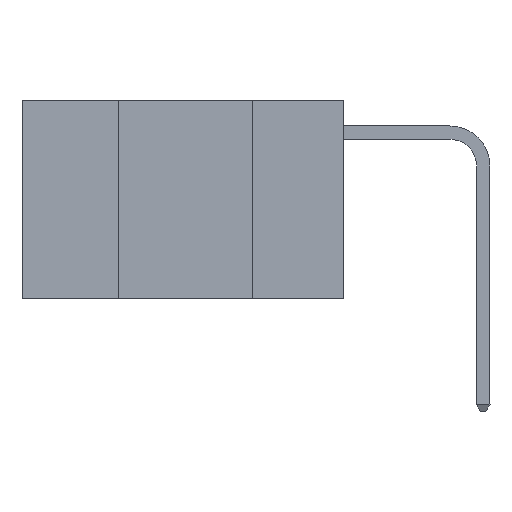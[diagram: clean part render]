
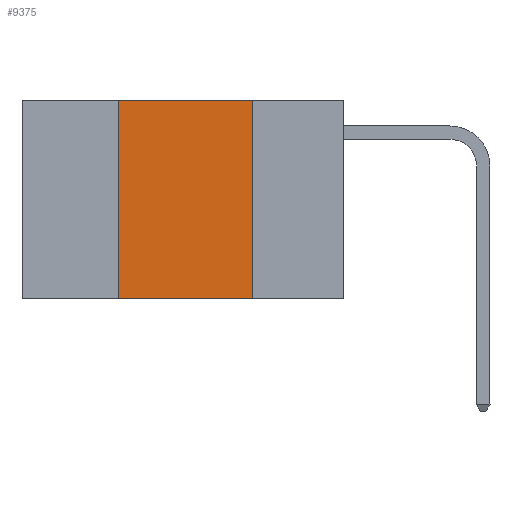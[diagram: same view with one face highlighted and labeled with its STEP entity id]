
A CAD part, left-side view. The second image highlights one B-rep face of the part: STEP entity #9375.
In plain terms, the highlighted planar face has unit normal (-1, 0, 0).
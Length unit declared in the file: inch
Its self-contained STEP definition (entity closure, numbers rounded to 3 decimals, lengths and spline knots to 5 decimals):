
#292 = ORIENTED_EDGE ( 'NONE', *, *, #7636, .T. ) ;
#629 = LINE ( 'NONE', #2177, #1024 ) ;
#890 = VECTOR ( 'NONE', #2272, 39.37008 ) ;
#930 = CARTESIAN_POINT ( 'NONE',  ( 0., 0.6, -0.37 ) ) ;
#1024 = VECTOR ( 'NONE', #1471, 39.37008 ) ;
#1281 = AXIS2_PLACEMENT_3D ( 'NONE', #4069, #4628, #7953 ) ;
#1471 = DIRECTION ( 'NONE',  ( 0., 0., 1. ) ) ;
#2177 = CARTESIAN_POINT ( 'NONE',  ( 0., 0.42, 0. ) ) ;
#2267 = VERTEX_POINT ( 'NONE', #10170 ) ;
#2272 = DIRECTION ( 'NONE',  ( 0., -1., 0. ) ) ;
#2513 = DIRECTION ( 'NONE',  ( 0., -1., 0. ) ) ;
#2635 = VERTEX_POINT ( 'NONE', #8420 ) ;
#2984 = VERTEX_POINT ( 'NONE', #5144 ) ;
#3816 = LINE ( 'NONE', #7000, #9246 ) ;
#4013 = FACE_OUTER_BOUND ( 'NONE', #5321, .T. ) ;
#4069 = CARTESIAN_POINT ( 'NONE',  ( 0., 0.6, 0. ) ) ;
#4628 = DIRECTION ( 'NONE',  ( 1., 0., 0. ) ) ;
#4758 = CARTESIAN_POINT ( 'NONE',  ( 0., 0.6, 0. ) ) ;
#5144 = CARTESIAN_POINT ( 'NONE',  ( 0., 0.17, 0. ) ) ;
#5321 = EDGE_LOOP ( 'NONE', ( #7345, #5951, #9402, #292 ) ) ;
#5951 = ORIENTED_EDGE ( 'NONE', *, *, #6680, .F. ) ;
#6680 = EDGE_CURVE ( 'NONE', #2267, #2984, #7622, .T. ) ;
#7000 = CARTESIAN_POINT ( 'NONE',  ( 0., 0.17, 0. ) ) ;
#7233 = PLANE ( 'NONE',  #1281 ) ;
#7345 = ORIENTED_EDGE ( 'NONE', *, *, #7482, .F. ) ;
#7482 = EDGE_CURVE ( 'NONE', #2984, #9340, #3816, .T. ) ;
#7578 = VECTOR ( 'NONE', #2513, 39.37008 ) ;
#7622 = LINE ( 'NONE', #4758, #890 ) ;
#7636 = EDGE_CURVE ( 'NONE', #2635, #9340, #9675, .T. ) ;
#7850 = EDGE_CURVE ( 'NONE', #2635, #2267, #629, .T. ) ;
#7953 = DIRECTION ( 'NONE',  ( 0., 0., -1. ) ) ;
#8420 = CARTESIAN_POINT ( 'NONE',  ( 0., 0.42, -0.37 ) ) ;
#8799 = CARTESIAN_POINT ( 'NONE',  ( 0., 0.17, -0.37 ) ) ;
#9246 = VECTOR ( 'NONE', #10047, 39.37008 ) ;
#9340 = VERTEX_POINT ( 'NONE', #8799 ) ;
#9375 = ADVANCED_FACE ( 'NONE', ( #4013 ), #7233, .F. ) ;
#9402 = ORIENTED_EDGE ( 'NONE', *, *, #7850, .F. ) ;
#9675 = LINE ( 'NONE', #930, #7578 ) ;
#10047 = DIRECTION ( 'NONE',  ( 0., 0., -1. ) ) ;
#10170 = CARTESIAN_POINT ( 'NONE',  ( 0., 0.42, 0. ) ) ;
